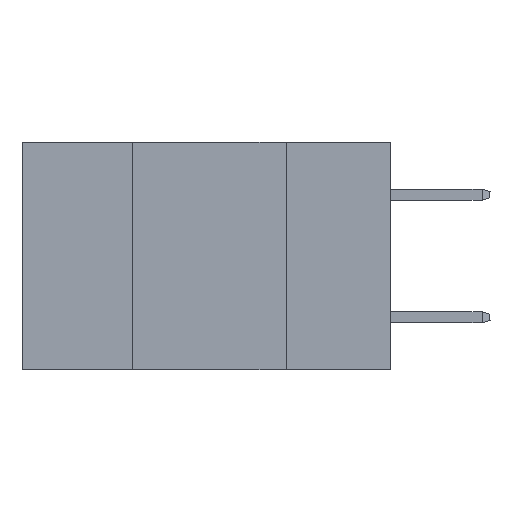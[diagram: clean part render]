
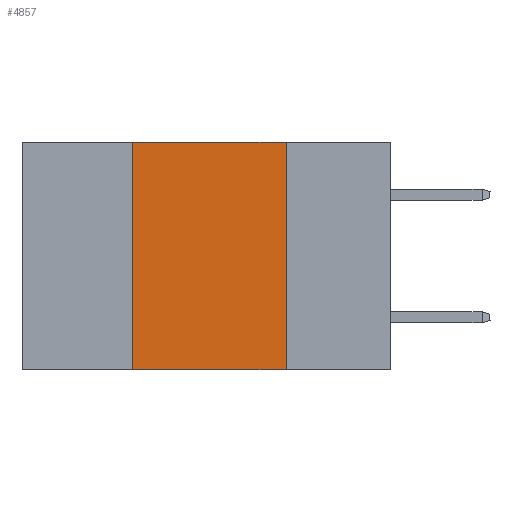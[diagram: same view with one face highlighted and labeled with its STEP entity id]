
A CAD part, left-side view. The second image highlights one B-rep face of the part: STEP entity #4857.
In plain terms, the highlighted planar face has unit normal (-1, 0, 0).
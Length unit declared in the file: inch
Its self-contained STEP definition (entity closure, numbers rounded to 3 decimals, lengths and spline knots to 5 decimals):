
#40 = CARTESIAN_POINT ( 'NONE',  ( 0., 0.42, 0. ) ) ;
#432 = LINE ( 'NONE', #10707, #8065 ) ;
#1666 = PLANE ( 'NONE',  #12792 ) ;
#2907 = ORIENTED_EDGE ( 'NONE', *, *, #15504, .F. ) ;
#3937 = ORIENTED_EDGE ( 'NONE', *, *, #11807, .F. ) ;
#4445 = ORIENTED_EDGE ( 'NONE', *, *, #15284, .T. ) ;
#4753 = VECTOR ( 'NONE', #7606, 39.37008 ) ;
#4810 = VERTEX_POINT ( 'NONE', #40 ) ;
#4821 = CARTESIAN_POINT ( 'NONE',  ( 0., 0.17, -0.37 ) ) ;
#4857 = ADVANCED_FACE ( 'NONE', ( #7629 ), #1666, .F. ) ;
#5452 = VECTOR ( 'NONE', #16615, 39.37008 ) ;
#5891 = VERTEX_POINT ( 'NONE', #19993 ) ;
#6029 = VERTEX_POINT ( 'NONE', #7933 ) ;
#6496 = VERTEX_POINT ( 'NONE', #4821 ) ;
#7520 = CARTESIAN_POINT ( 'NONE',  ( 0., 0.17, 0. ) ) ;
#7606 = DIRECTION ( 'NONE',  ( 0., -1., 0. ) ) ;
#7629 = FACE_OUTER_BOUND ( 'NONE', #20025, .T. ) ;
#7933 = CARTESIAN_POINT ( 'NONE',  ( 0., 0.17, 0. ) ) ;
#8065 = VECTOR ( 'NONE', #16716, 39.37008 ) ;
#8142 = DIRECTION ( 'NONE',  ( 0., -1., 0. ) ) ;
#8192 = VECTOR ( 'NONE', #8142, 39.37008 ) ;
#10461 = CARTESIAN_POINT ( 'NONE',  ( 0., 0.6, 0. ) ) ;
#10707 = CARTESIAN_POINT ( 'NONE',  ( 0., 0.42, 0. ) ) ;
#11807 = EDGE_CURVE ( 'NONE', #5891, #4810, #432, .T. ) ;
#12137 = CARTESIAN_POINT ( 'NONE',  ( 0., 0.6, -0.37 ) ) ;
#12792 = AXIS2_PLACEMENT_3D ( 'NONE', #10461, #15420, #14449 ) ;
#14119 = LINE ( 'NONE', #7520, #5452 ) ;
#14449 = DIRECTION ( 'NONE',  ( 0., 0., -1. ) ) ;
#15284 = EDGE_CURVE ( 'NONE', #5891, #6496, #17924, .T. ) ;
#15420 = DIRECTION ( 'NONE',  ( 1., 0., 0. ) ) ;
#15504 = EDGE_CURVE ( 'NONE', #4810, #6029, #16278, .T. ) ;
#15908 = EDGE_CURVE ( 'NONE', #6029, #6496, #14119, .T. ) ;
#16278 = LINE ( 'NONE', #16836, #8192 ) ;
#16615 = DIRECTION ( 'NONE',  ( 0., 0., -1. ) ) ;
#16716 = DIRECTION ( 'NONE',  ( 0., 0., 1. ) ) ;
#16836 = CARTESIAN_POINT ( 'NONE',  ( 0., 0.6, 0. ) ) ;
#17924 = LINE ( 'NONE', #12137, #4753 ) ;
#18325 = ORIENTED_EDGE ( 'NONE', *, *, #15908, .F. ) ;
#19993 = CARTESIAN_POINT ( 'NONE',  ( 0., 0.42, -0.37 ) ) ;
#20025 = EDGE_LOOP ( 'NONE', ( #18325, #2907, #3937, #4445 ) ) ;
